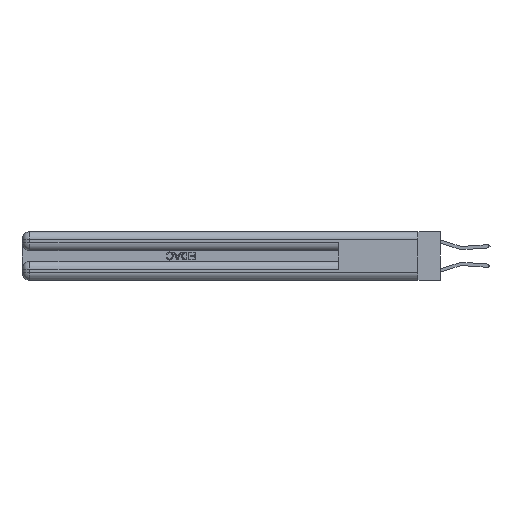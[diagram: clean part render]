
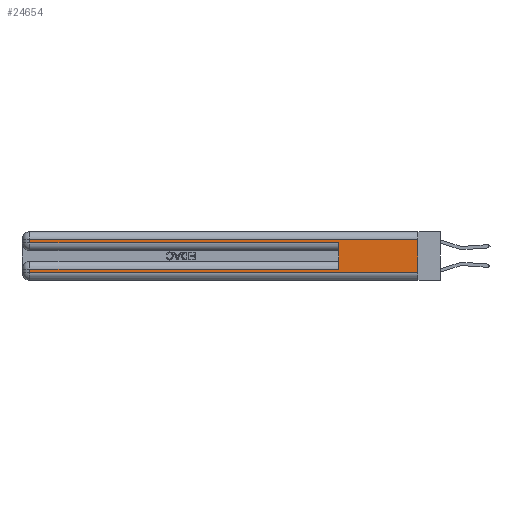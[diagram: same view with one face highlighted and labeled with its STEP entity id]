
A CAD part, left-side view. The second image highlights one B-rep face of the part: STEP entity #24654.
In plain terms, the highlighted planar face has unit normal (-1, 0, 0).
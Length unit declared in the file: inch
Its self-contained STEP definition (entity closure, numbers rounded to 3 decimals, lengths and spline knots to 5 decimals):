
#288 = LINE ( 'NONE', #12833, #7547 ) ;
#870 = EDGE_CURVE ( 'NONE', #4088, #2777, #32248, .T. ) ;
#1427 = VECTOR ( 'NONE', #19469, 39.37008 ) ;
#1880 = VECTOR ( 'NONE', #13232, 39.37008 ) ;
#2223 = CARTESIAN_POINT ( 'NONE',  ( 0., 2.94, 0.37 ) ) ;
#2777 = VERTEX_POINT ( 'NONE', #14074 ) ;
#3406 = VECTOR ( 'NONE', #25416, 39.37008 ) ;
#3427 = ORIENTED_EDGE ( 'NONE', *, *, #22160, .F. ) ;
#4088 = VERTEX_POINT ( 'NONE', #4187 ) ;
#4187 = CARTESIAN_POINT ( 'NONE',  ( 0., 2.94, 0.285 ) ) ;
#4396 = CARTESIAN_POINT ( 'NONE',  ( 0., 2.94, 0.37 ) ) ;
#5030 = VERTEX_POINT ( 'NONE', #10833 ) ;
#5069 = CARTESIAN_POINT ( 'NONE',  ( 0., 0., 0.37 ) ) ;
#5779 = ORIENTED_EDGE ( 'NONE', *, *, #870, .T. ) ;
#6210 = AXIS2_PLACEMENT_3D ( 'NONE', #14407, #25411, #8996 ) ;
#6257 = PLANE ( 'NONE',  #6210 ) ;
#7304 = DIRECTION ( 'NONE',  ( 0., -1., 0. ) ) ;
#7467 = VERTEX_POINT ( 'NONE', #13328 ) ;
#7547 = VECTOR ( 'NONE', #7304, 39.37008 ) ;
#7910 = EDGE_CURVE ( 'NONE', #10000, #13191, #288, .T. ) ;
#8996 = DIRECTION ( 'NONE',  ( 0., 0., -1. ) ) ;
#10000 = VERTEX_POINT ( 'NONE', #24268 ) ;
#10032 = ORIENTED_EDGE ( 'NONE', *, *, #32054, .T. ) ;
#10686 = LINE ( 'NONE', #5069, #33384 ) ;
#10833 = CARTESIAN_POINT ( 'NONE',  ( 0., 2.94, 0.085 ) ) ;
#11147 = LINE ( 'NONE', #23733, #15840 ) ;
#12248 = CARTESIAN_POINT ( 'NONE',  ( 0., 0., 0.06 ) ) ;
#12614 = EDGE_CURVE ( 'NONE', #23784, #4088, #13646, .T. ) ;
#12833 = CARTESIAN_POINT ( 'NONE',  ( 0., 0., 0.06 ) ) ;
#12883 = ORIENTED_EDGE ( 'NONE', *, *, #12614, .T. ) ;
#13191 = VERTEX_POINT ( 'NONE', #12248 ) ;
#13232 = DIRECTION ( 'NONE',  ( 0., 0., -1. ) ) ;
#13328 = CARTESIAN_POINT ( 'NONE',  ( 0., 0., 0.31 ) ) ;
#13646 = LINE ( 'NONE', #4396, #33770 ) ;
#14074 = CARTESIAN_POINT ( 'NONE',  ( 0., 0.6, 0.285 ) ) ;
#14407 = CARTESIAN_POINT ( 'NONE',  ( 0., 0., 0.37 ) ) ;
#14444 = EDGE_CURVE ( 'NONE', #33660, #2777, #30930, .T. ) ;
#14852 = FACE_OUTER_BOUND ( 'NONE', #24635, .T. ) ;
#15283 = DIRECTION ( 'NONE',  ( 0., 0., -1. ) ) ;
#15840 = VECTOR ( 'NONE', #34733, 39.37008 ) ;
#16323 = EDGE_CURVE ( 'NONE', #33660, #5030, #25248, .T. ) ;
#16379 = VECTOR ( 'NONE', #23190, 39.37008 ) ;
#16427 = LINE ( 'NONE', #2223, #1880 ) ;
#16716 = CARTESIAN_POINT ( 'NONE',  ( 0., 0., 0.285 ) ) ;
#19349 = CARTESIAN_POINT ( 'NONE',  ( 0., 0.6, 0.085 ) ) ;
#19469 = DIRECTION ( 'NONE',  ( 0., -1., 0. ) ) ;
#20444 = CARTESIAN_POINT ( 'NONE',  ( 0., 0.6, 0.145 ) ) ;
#22160 = EDGE_CURVE ( 'NONE', #7467, #13191, #10686, .T. ) ;
#22406 = ORIENTED_EDGE ( 'NONE', *, *, #29882, .T. ) ;
#22672 = CARTESIAN_POINT ( 'NONE',  ( 0., 0., 0.085 ) ) ;
#23190 = DIRECTION ( 'NONE',  ( 0., 0., 1. ) ) ;
#23560 = ORIENTED_EDGE ( 'NONE', *, *, #16323, .T. ) ;
#23733 = CARTESIAN_POINT ( 'NONE',  ( 0., 0., 0.31 ) ) ;
#23784 = VERTEX_POINT ( 'NONE', #26025 ) ;
#24268 = CARTESIAN_POINT ( 'NONE',  ( 0., 2.94, 0.06 ) ) ;
#24635 = EDGE_LOOP ( 'NONE', ( #3427, #10032, #12883, #5779, #26955, #23560, #22406, #31630 ) ) ;
#24654 = ADVANCED_FACE ( 'NONE', ( #14852 ), #6257, .F. ) ;
#25248 = LINE ( 'NONE', #22672, #3406 ) ;
#25411 = DIRECTION ( 'NONE',  ( 1., 0., 0. ) ) ;
#25416 = DIRECTION ( 'NONE',  ( 0., 1., 0. ) ) ;
#26025 = CARTESIAN_POINT ( 'NONE',  ( 0., 2.94, 0.31 ) ) ;
#26955 = ORIENTED_EDGE ( 'NONE', *, *, #14444, .F. ) ;
#26967 = DIRECTION ( 'NONE',  ( 0., 0., -1. ) ) ;
#29882 = EDGE_CURVE ( 'NONE', #5030, #10000, #16427, .T. ) ;
#30930 = LINE ( 'NONE', #20444, #16379 ) ;
#31630 = ORIENTED_EDGE ( 'NONE', *, *, #7910, .T. ) ;
#32054 = EDGE_CURVE ( 'NONE', #7467, #23784, #11147, .T. ) ;
#32248 = LINE ( 'NONE', #16716, #1427 ) ;
#33384 = VECTOR ( 'NONE', #26967, 39.37008 ) ;
#33660 = VERTEX_POINT ( 'NONE', #19349 ) ;
#33770 = VECTOR ( 'NONE', #15283, 39.37008 ) ;
#34733 = DIRECTION ( 'NONE',  ( 0., 1., 0. ) ) ;
